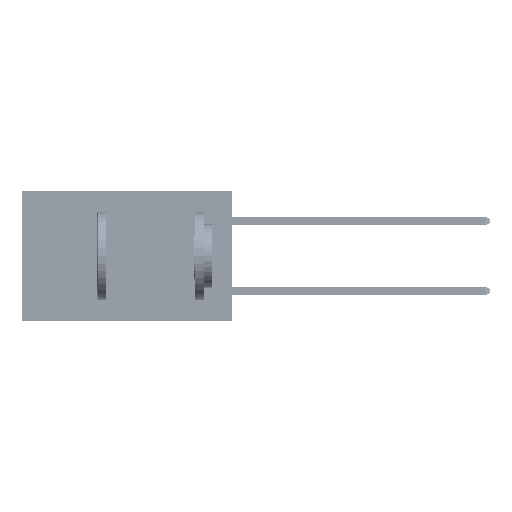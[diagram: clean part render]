
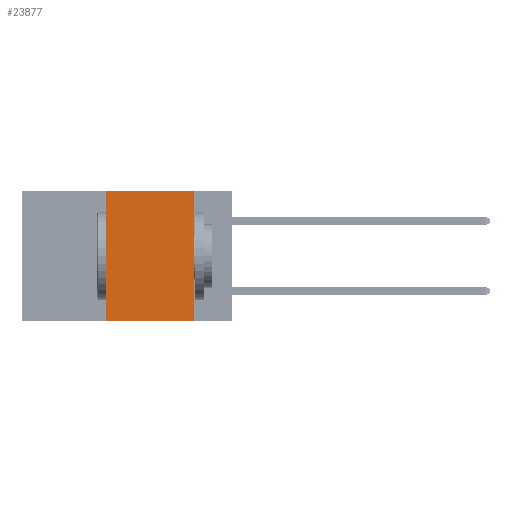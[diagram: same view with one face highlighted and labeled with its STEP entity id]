
A CAD part, left-side view. The second image highlights one B-rep face of the part: STEP entity #23877.
In plain terms, the highlighted planar face has unit normal (-1, 0, 0).
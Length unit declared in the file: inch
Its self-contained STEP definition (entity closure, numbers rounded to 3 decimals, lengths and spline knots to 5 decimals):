
#1570 = VECTOR ( 'NONE', #11320, 39.37008 ) ;
#1888 = EDGE_LOOP ( 'NONE', ( #48558, #45570, #27300, #12190 ) ) ;
#3575 = AXIS2_PLACEMENT_3D ( 'NONE', #29146, #13940, #33004 ) ;
#4305 = LINE ( 'NONE', #22623, #30689 ) ;
#5112 = VERTEX_POINT ( 'NONE', #34894 ) ;
#10269 = PLANE ( 'NONE',  #3575 ) ;
#10399 = VERTEX_POINT ( 'NONE', #39877 ) ;
#11320 = DIRECTION ( 'NONE',  ( 0., -1., 0. ) ) ;
#12190 = ORIENTED_EDGE ( 'NONE', *, *, #29545, .T. ) ;
#13940 = DIRECTION ( 'NONE',  ( 1., 0., 0. ) ) ;
#17365 = DIRECTION ( 'NONE',  ( 0., -1., 0. ) ) ;
#21537 = EDGE_CURVE ( 'NONE', #27099, #10399, #4305, .T. ) ;
#22623 = CARTESIAN_POINT ( 'NONE',  ( 0., 0.36, 0. ) ) ;
#23744 = LINE ( 'NONE', #31427, #27349 ) ;
#23877 = ADVANCED_FACE ( 'NONE', ( #27448 ), #10269, .F. ) ;
#25027 = EDGE_CURVE ( 'NONE', #10399, #5112, #23744, .T. ) ;
#26352 = VERTEX_POINT ( 'NONE', #37354 ) ;
#27099 = VERTEX_POINT ( 'NONE', #45933 ) ;
#27300 = ORIENTED_EDGE ( 'NONE', *, *, #21537, .F. ) ;
#27349 = VECTOR ( 'NONE', #17365, 39.37008 ) ;
#27448 = FACE_OUTER_BOUND ( 'NONE', #1888, .T. ) ;
#28114 = LINE ( 'NONE', #35399, #47179 ) ;
#29146 = CARTESIAN_POINT ( 'NONE',  ( 0., 0.6, 0. ) ) ;
#29545 = EDGE_CURVE ( 'NONE', #27099, #26352, #36796, .T. ) ;
#29864 = CARTESIAN_POINT ( 'NONE',  ( 0., 0.6, -0.37 ) ) ;
#30689 = VECTOR ( 'NONE', #41984, 39.37008 ) ;
#31427 = CARTESIAN_POINT ( 'NONE',  ( 0., 0.6, 0. ) ) ;
#33004 = DIRECTION ( 'NONE',  ( 0., 0., -1. ) ) ;
#33937 = EDGE_CURVE ( 'NONE', #5112, #26352, #28114, .T. ) ;
#34894 = CARTESIAN_POINT ( 'NONE',  ( 0., 0.11, 0. ) ) ;
#35399 = CARTESIAN_POINT ( 'NONE',  ( 0., 0.11, 0. ) ) ;
#36796 = LINE ( 'NONE', #29864, #1570 ) ;
#37354 = CARTESIAN_POINT ( 'NONE',  ( 0., 0.11, -0.37 ) ) ;
#37936 = DIRECTION ( 'NONE',  ( 0., 0., -1. ) ) ;
#39877 = CARTESIAN_POINT ( 'NONE',  ( 0., 0.36, 0. ) ) ;
#41984 = DIRECTION ( 'NONE',  ( 0., 0., 1. ) ) ;
#45570 = ORIENTED_EDGE ( 'NONE', *, *, #25027, .F. ) ;
#45933 = CARTESIAN_POINT ( 'NONE',  ( 0., 0.36, -0.37 ) ) ;
#47179 = VECTOR ( 'NONE', #37936, 39.37008 ) ;
#48558 = ORIENTED_EDGE ( 'NONE', *, *, #33937, .F. ) ;
